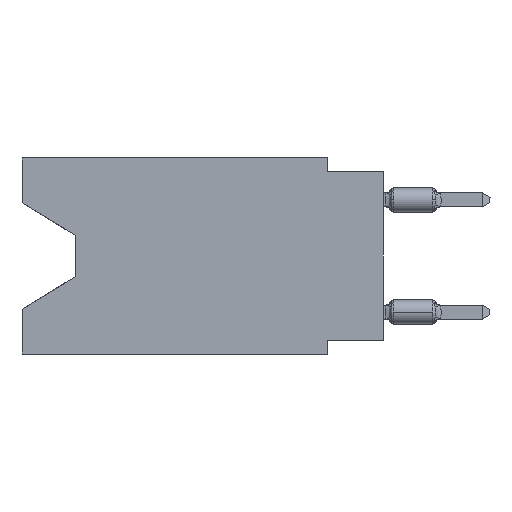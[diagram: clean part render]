
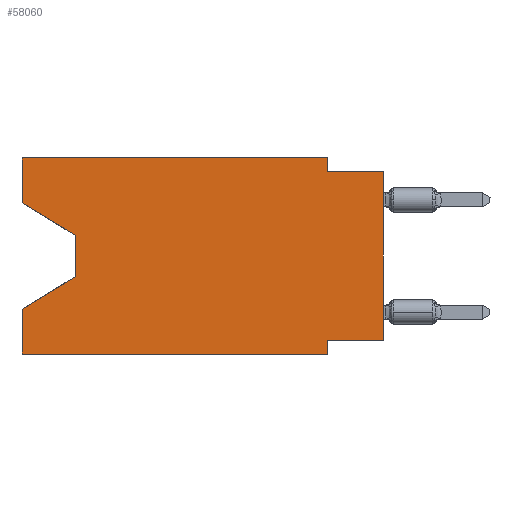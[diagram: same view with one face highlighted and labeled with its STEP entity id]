
A CAD part, left-side view. The second image highlights one B-rep face of the part: STEP entity #58060.
In plain terms, the highlighted planar face has unit normal (-1, 0, 0).
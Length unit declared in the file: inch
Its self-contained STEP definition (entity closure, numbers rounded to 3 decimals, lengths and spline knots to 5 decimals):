
#229 = CARTESIAN_POINT ( 'NONE',  ( 0., 0.645, 0. ) ) ;
#778 = ORIENTED_EDGE ( 'NONE', *, *, #55844, .T. ) ;
#1349 = DIRECTION ( 'NONE',  ( 1., 0., 0. ) ) ;
#1944 = FACE_OUTER_BOUND ( 'NONE', #2987, .T. ) ;
#2857 = LINE ( 'NONE', #7981, #28002 ) ;
#2987 = EDGE_LOOP ( 'NONE', ( #48189, #11592, #30778, #15889, #778, #23989, #20361, #32351, #13767, #39825, #4527, #38886 ) ) ;
#3737 = VECTOR ( 'NONE', #22929, 39.37008 ) ;
#3864 = DIRECTION ( 'NONE',  ( 0., 1., 0. ) ) ;
#4527 = ORIENTED_EDGE ( 'NONE', *, *, #48974, .F. ) ;
#4734 = DIRECTION ( 'NONE',  ( 0., -1., 0. ) ) ;
#5277 = VERTEX_POINT ( 'NONE', #37031 ) ;
#5318 = VECTOR ( 'NONE', #3864, 39.37008 ) ;
#5784 = VERTEX_POINT ( 'NONE', #27936 ) ;
#5839 = VECTOR ( 'NONE', #20743, 39.37008 ) ;
#7182 = VECTOR ( 'NONE', #4734, 39.37008 ) ;
#7981 = CARTESIAN_POINT ( 'NONE',  ( 0., 0., -0.025 ) ) ;
#8435 = DIRECTION ( 'NONE',  ( 0., 0., 1. ) ) ;
#8747 = LINE ( 'NONE', #46003, #42053 ) ;
#11227 = EDGE_CURVE ( 'NONE', #22802, #36598, #2857, .T. ) ;
#11521 = CARTESIAN_POINT ( 'NONE',  ( 0., 0.1, -0.325 ) ) ;
#11592 = ORIENTED_EDGE ( 'NONE', *, *, #55553, .T. ) ;
#12868 = VERTEX_POINT ( 'NONE', #56723 ) ;
#13647 = LINE ( 'NONE', #41283, #57617 ) ;
#13767 = ORIENTED_EDGE ( 'NONE', *, *, #11227, .F. ) ;
#15704 = CARTESIAN_POINT ( 'NONE',  ( 0., 0.1, -0.025 ) ) ;
#15889 = ORIENTED_EDGE ( 'NONE', *, *, #56321, .F. ) ;
#16145 = CARTESIAN_POINT ( 'NONE',  ( 0., 0.1, 0. ) ) ;
#18194 = VECTOR ( 'NONE', #18574, 39.37008 ) ;
#18574 = DIRECTION ( 'NONE',  ( 0., 0., 1. ) ) ;
#20361 = ORIENTED_EDGE ( 'NONE', *, *, #50051, .F. ) ;
#20743 = DIRECTION ( 'NONE',  ( 0., 0., 1. ) ) ;
#21095 = LINE ( 'NONE', #58671, #53665 ) ;
#21285 = DIRECTION ( 'NONE',  ( 0., 0., -1. ) ) ;
#21297 = EDGE_CURVE ( 'NONE', #38628, #12868, #8747, .T. ) ;
#21523 = VERTEX_POINT ( 'NONE', #30033 ) ;
#21968 = CARTESIAN_POINT ( 'NONE',  ( 0., 0.645, 0. ) ) ;
#22266 = LINE ( 'NONE', #21968, #47417 ) ;
#22620 = CARTESIAN_POINT ( 'NONE',  ( 0., 0.55, -0.138 ) ) ;
#22663 = LINE ( 'NONE', #32277, #26729 ) ;
#22802 = VERTEX_POINT ( 'NONE', #15704 ) ;
#22929 = DIRECTION ( 'NONE',  ( 0., 0., -1. ) ) ;
#23430 = EDGE_CURVE ( 'NONE', #39905, #23560, #13647, .T. ) ;
#23560 = VERTEX_POINT ( 'NONE', #56616 ) ;
#23989 = ORIENTED_EDGE ( 'NONE', *, *, #53629, .F. ) ;
#24044 = EDGE_CURVE ( 'NONE', #5784, #36598, #25840, .T. ) ;
#24807 = VERTEX_POINT ( 'NONE', #42254 ) ;
#25691 = DIRECTION ( 'NONE',  ( 0., -1., 0. ) ) ;
#25840 = LINE ( 'NONE', #49297, #5839 ) ;
#26729 = VECTOR ( 'NONE', #21285, 39.37008 ) ;
#27423 = LINE ( 'NONE', #22620, #3737 ) ;
#27936 = CARTESIAN_POINT ( 'NONE',  ( 0., 0., -0.325 ) ) ;
#28002 = VECTOR ( 'NONE', #25691, 39.37008 ) ;
#28410 = DIRECTION ( 'NONE',  ( 0., 0., -1. ) ) ;
#30033 = CARTESIAN_POINT ( 'NONE',  ( 0., 0.1, -0.35 ) ) ;
#30778 = ORIENTED_EDGE ( 'NONE', *, *, #23430, .T. ) ;
#32277 = CARTESIAN_POINT ( 'NONE',  ( 0., 0.1, -0.35 ) ) ;
#32351 = ORIENTED_EDGE ( 'NONE', *, *, #24044, .T. ) ;
#32388 = LINE ( 'NONE', #229, #18194 ) ;
#32936 = CARTESIAN_POINT ( 'NONE',  ( 0., 0.645, 0. ) ) ;
#35803 = DIRECTION ( 'NONE',  ( 0., -1., 0. ) ) ;
#36598 = VERTEX_POINT ( 'NONE', #53387 ) ;
#36896 = LINE ( 'NONE', #46803, #7182 ) ;
#36982 = DIRECTION ( 'NONE',  ( 0., -0.855, -0.519 ) ) ;
#37031 = CARTESIAN_POINT ( 'NONE',  ( 0., 0.645, -0.35 ) ) ;
#37736 = DIRECTION ( 'NONE',  ( 0., 0., -1. ) ) ;
#38628 = VERTEX_POINT ( 'NONE', #59330 ) ;
#38886 = ORIENTED_EDGE ( 'NONE', *, *, #48412, .F. ) ;
#39825 = ORIENTED_EDGE ( 'NONE', *, *, #50744, .F. ) ;
#39905 = VERTEX_POINT ( 'NONE', #50314 ) ;
#40243 = CARTESIAN_POINT ( 'NONE',  ( 0., 0., -0.325 ) ) ;
#41283 = CARTESIAN_POINT ( 'NONE',  ( 0., 0.55, -0.212 ) ) ;
#41877 = VECTOR ( 'NONE', #37736, 39.37008 ) ;
#42053 = VECTOR ( 'NONE', #36982, 39.37008 ) ;
#42254 = CARTESIAN_POINT ( 'NONE',  ( 0., 0.645, 0. ) ) ;
#42300 = AXIS2_PLACEMENT_3D ( 'NONE', #32936, #1349, #28410 ) ;
#46003 = CARTESIAN_POINT ( 'NONE',  ( 0., 0.645, -0.08025 ) ) ;
#46747 = PLANE ( 'NONE',  #42300 ) ;
#46803 = CARTESIAN_POINT ( 'NONE',  ( 0., 0.645, 0. ) ) ;
#47417 = VECTOR ( 'NONE', #8435, 39.37008 ) ;
#48189 = ORIENTED_EDGE ( 'NONE', *, *, #21297, .T. ) ;
#48242 = LINE ( 'NONE', #57261, #41877 ) ;
#48412 = EDGE_CURVE ( 'NONE', #38628, #24807, #22266, .T. ) ;
#48974 = EDGE_CURVE ( 'NONE', #24807, #57753, #36896, .T. ) ;
#49297 = CARTESIAN_POINT ( 'NONE',  ( 0., 0., 0. ) ) ;
#49866 = LINE ( 'NONE', #40243, #5318 ) ;
#50051 = EDGE_CURVE ( 'NONE', #5784, #59456, #49866, .T. ) ;
#50314 = CARTESIAN_POINT ( 'NONE',  ( 0., 0.55, -0.212 ) ) ;
#50744 = EDGE_CURVE ( 'NONE', #57753, #22802, #48242, .T. ) ;
#53387 = CARTESIAN_POINT ( 'NONE',  ( 0., 0., -0.025 ) ) ;
#53629 = EDGE_CURVE ( 'NONE', #59456, #21523, #22663, .T. ) ;
#53665 = VECTOR ( 'NONE', #35803, 39.37008 ) ;
#55425 = DIRECTION ( 'NONE',  ( 0., 0.855, -0.519 ) ) ;
#55553 = EDGE_CURVE ( 'NONE', #12868, #39905, #27423, .T. ) ;
#55844 = EDGE_CURVE ( 'NONE', #5277, #21523, #21095, .T. ) ;
#56321 = EDGE_CURVE ( 'NONE', #5277, #23560, #32388, .T. ) ;
#56616 = CARTESIAN_POINT ( 'NONE',  ( 0., 0.645, -0.26975 ) ) ;
#56723 = CARTESIAN_POINT ( 'NONE',  ( 0., 0.55, -0.138 ) ) ;
#57261 = CARTESIAN_POINT ( 'NONE',  ( 0., 0.1, 0. ) ) ;
#57617 = VECTOR ( 'NONE', #55425, 39.37008 ) ;
#57753 = VERTEX_POINT ( 'NONE', #16145 ) ;
#58060 = ADVANCED_FACE ( 'NONE', ( #1944 ), #46747, .F. ) ;
#58671 = CARTESIAN_POINT ( 'NONE',  ( 0., 0.645, -0.35 ) ) ;
#59330 = CARTESIAN_POINT ( 'NONE',  ( 0., 0.645, -0.08025 ) ) ;
#59456 = VERTEX_POINT ( 'NONE', #11521 ) ;
